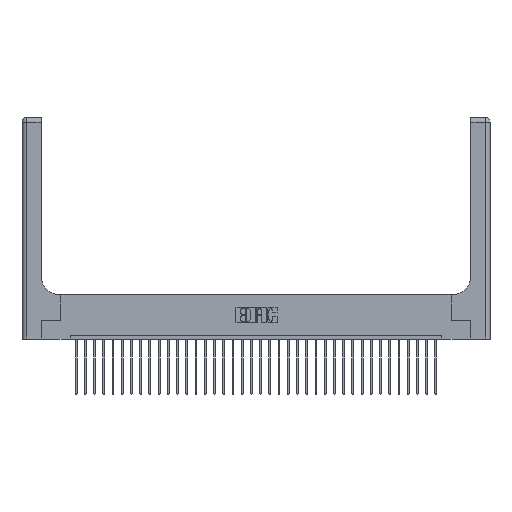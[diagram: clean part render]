
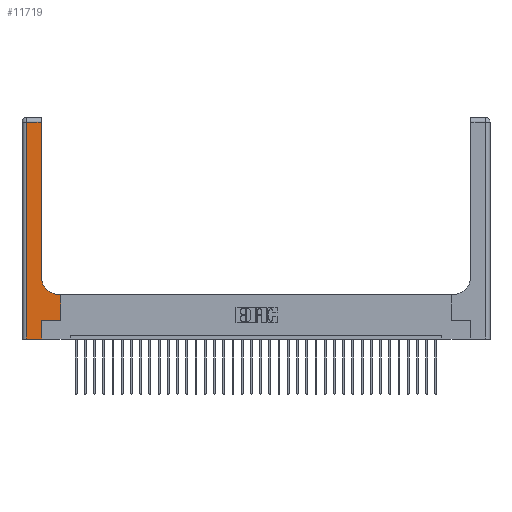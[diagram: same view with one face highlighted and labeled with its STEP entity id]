
A CAD part, top view. The second image highlights one B-rep face of the part: STEP entity #11719.
In plain terms, the highlighted planar face has unit normal (0, 0, 1).
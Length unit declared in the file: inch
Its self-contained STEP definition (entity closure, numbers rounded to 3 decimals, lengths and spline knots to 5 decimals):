
#221 = CARTESIAN_POINT ( 'NONE',  ( 0.51, 0.6, 0.37 ) ) ;
#793 = CARTESIAN_POINT ( 'NONE',  ( 0.265, 0.25, 0.37 ) ) ;
#1104 = ORIENTED_EDGE ( 'NONE', *, *, #22121, .T. ) ;
#1145 = CARTESIAN_POINT ( 'NONE',  ( 0.06, 0., 0.37 ) ) ;
#1183 = ORIENTED_EDGE ( 'NONE', *, *, #2041, .T. ) ;
#1830 = VECTOR ( 'NONE', #4632, 39.37008 ) ;
#1979 = CARTESIAN_POINT ( 'NONE',  ( 0.528, 0.25, 0.37 ) ) ;
#2041 = EDGE_CURVE ( 'NONE', #20420, #25706, #7447, .T. ) ;
#2274 = CARTESIAN_POINT ( 'NONE',  ( 0.26, 3., 0.37 ) ) ;
#2281 = VERTEX_POINT ( 'NONE', #13493 ) ;
#2523 = ORIENTED_EDGE ( 'NONE', *, *, #25333, .T. ) ;
#2787 = DIRECTION ( 'NONE',  ( -1., 0., 0. ) ) ;
#2920 = CARTESIAN_POINT ( 'NONE',  ( 0.265, 0., 0.37 ) ) ;
#3052 = VECTOR ( 'NONE', #29563, 39.37008 ) ;
#3613 = VERTEX_POINT ( 'NONE', #11923 ) ;
#3988 = VERTEX_POINT ( 'NONE', #221 ) ;
#4012 = LINE ( 'NONE', #1979, #16542 ) ;
#4213 = CARTESIAN_POINT ( 'NONE',  ( 0.528, 0.25, 0.37 ) ) ;
#4587 = EDGE_CURVE ( 'NONE', #9907, #2281, #13792, .T. ) ;
#4632 = DIRECTION ( 'NONE',  ( 0., 1., 0. ) ) ;
#5730 = DIRECTION ( 'NONE',  ( 0., 1., 0. ) ) ;
#7447 = LINE ( 'NONE', #2920, #15947 ) ;
#7451 = DIRECTION ( 'NONE',  ( 1., 0., 0. ) ) ;
#7624 = LINE ( 'NONE', #14917, #15998 ) ;
#7802 = VERTEX_POINT ( 'NONE', #4213 ) ;
#7964 = EDGE_CURVE ( 'NONE', #3988, #9907, #13284, .T. ) ;
#7984 = ORIENTED_EDGE ( 'NONE', *, *, #7964, .T. ) ;
#8372 = LINE ( 'NONE', #27817, #10957 ) ;
#9066 = VERTEX_POINT ( 'NONE', #1145 ) ;
#9648 = CARTESIAN_POINT ( 'NONE',  ( 0.51, 0.85, 0.37 ) ) ;
#9907 = VERTEX_POINT ( 'NONE', #25295 ) ;
#9997 = AXIS2_PLACEMENT_3D ( 'NONE', #13110, #22612, #17936 ) ;
#10778 = EDGE_CURVE ( 'NONE', #3613, #9066, #8372, .T. ) ;
#10957 = VECTOR ( 'NONE', #13179, 39.37008 ) ;
#11620 = VERTEX_POINT ( 'NONE', #22766 ) ;
#11719 = ADVANCED_FACE ( 'NONE', ( #12957 ), #27586, .F. ) ;
#11923 = CARTESIAN_POINT ( 'NONE',  ( 0.06, 2.94, 0.37 ) ) ;
#12438 = EDGE_CURVE ( 'NONE', #2281, #3613, #7624, .T. ) ;
#12957 = FACE_OUTER_BOUND ( 'NONE', #14842, .T. ) ;
#13110 = CARTESIAN_POINT ( 'NONE',  ( 0., 3., 0.37 ) ) ;
#13179 = DIRECTION ( 'NONE',  ( 0., -1., 0. ) ) ;
#13284 = CIRCLE ( 'NONE', #14855, 0.25 ) ;
#13493 = CARTESIAN_POINT ( 'NONE',  ( 0.26, 2.94, 0.37 ) ) ;
#13792 = LINE ( 'NONE', #2274, #1830 ) ;
#14714 = CARTESIAN_POINT ( 'NONE',  ( 0.265, 0.25, 0.37 ) ) ;
#14842 = EDGE_LOOP ( 'NONE', ( #27548, #30687, #20414, #17456, #1183, #1104, #2523, #15582, #7984 ) ) ;
#14855 = AXIS2_PLACEMENT_3D ( 'NONE', #9648, #19418, #7451 ) ;
#14917 = CARTESIAN_POINT ( 'NONE',  ( 0., 2.94, 0.37 ) ) ;
#15582 = ORIENTED_EDGE ( 'NONE', *, *, #26752, .T. ) ;
#15947 = VECTOR ( 'NONE', #5730, 39.37008 ) ;
#15998 = VECTOR ( 'NONE', #2787, 39.37008 ) ;
#16542 = VECTOR ( 'NONE', #20653, 39.37008 ) ;
#16576 = LINE ( 'NONE', #26062, #17100 ) ;
#16696 = CARTESIAN_POINT ( 'NONE',  ( 0., 0., 0.37 ) ) ;
#17100 = VECTOR ( 'NONE', #18749, 39.37008 ) ;
#17456 = ORIENTED_EDGE ( 'NONE', *, *, #29926, .T. ) ;
#17936 = DIRECTION ( 'NONE',  ( -1., 0., 0. ) ) ;
#18749 = DIRECTION ( 'NONE',  ( -1., 0., 0. ) ) ;
#19418 = DIRECTION ( 'NONE',  ( 0., 0., -1. ) ) ;
#19711 = VECTOR ( 'NONE', #30683, 39.37008 ) ;
#20414 = ORIENTED_EDGE ( 'NONE', *, *, #10778, .T. ) ;
#20420 = VERTEX_POINT ( 'NONE', #23211 ) ;
#20653 = DIRECTION ( 'NONE',  ( 0., 1., 0. ) ) ;
#22121 = EDGE_CURVE ( 'NONE', #25706, #7802, #29109, .T. ) ;
#22612 = DIRECTION ( 'NONE',  ( 0., 0., -1. ) ) ;
#22766 = CARTESIAN_POINT ( 'NONE',  ( 0.528, 0.6, 0.37 ) ) ;
#23211 = CARTESIAN_POINT ( 'NONE',  ( 0.265, 0., 0.37 ) ) ;
#25295 = CARTESIAN_POINT ( 'NONE',  ( 0.26, 0.85, 0.37 ) ) ;
#25333 = EDGE_CURVE ( 'NONE', #7802, #11620, #4012, .T. ) ;
#25706 = VERTEX_POINT ( 'NONE', #14714 ) ;
#26062 = CARTESIAN_POINT ( 'NONE',  ( 0.26, 0.6, 0.37 ) ) ;
#26752 = EDGE_CURVE ( 'NONE', #11620, #3988, #16576, .T. ) ;
#27548 = ORIENTED_EDGE ( 'NONE', *, *, #4587, .T. ) ;
#27586 = PLANE ( 'NONE',  #9997 ) ;
#27817 = CARTESIAN_POINT ( 'NONE',  ( 0.06, 3., 0.37 ) ) ;
#28366 = LINE ( 'NONE', #16696, #19711 ) ;
#29109 = LINE ( 'NONE', #793, #3052 ) ;
#29563 = DIRECTION ( 'NONE',  ( 1., 0., 0. ) ) ;
#29926 = EDGE_CURVE ( 'NONE', #9066, #20420, #28366, .T. ) ;
#30683 = DIRECTION ( 'NONE',  ( 1., 0., 0. ) ) ;
#30687 = ORIENTED_EDGE ( 'NONE', *, *, #12438, .T. ) ;
